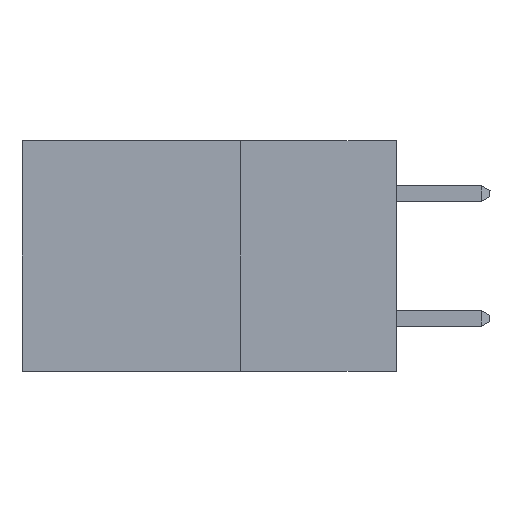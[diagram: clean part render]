
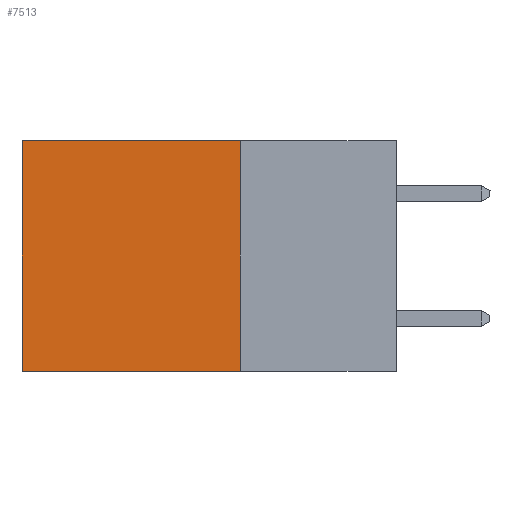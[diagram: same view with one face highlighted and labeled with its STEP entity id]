
A CAD part, left-side view. The second image highlights one B-rep face of the part: STEP entity #7513.
In plain terms, the highlighted planar face has unit normal (-1, 0, 0).
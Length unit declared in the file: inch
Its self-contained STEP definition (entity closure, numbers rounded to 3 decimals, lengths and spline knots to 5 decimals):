
#2 = CARTESIAN_POINT ( 'NONE',  ( 0.298, 0.25, 0. ) ) ;
#281 = FACE_OUTER_BOUND ( 'NONE', #5982, .T. ) ;
#2840 = LINE ( 'NONE', #5023, #15257 ) ;
#3210 = LINE ( 'NONE', #6717, #11351 ) ;
#3358 = ORIENTED_EDGE ( 'NONE', *, *, #16351, .T. ) ;
#3362 = EDGE_CURVE ( 'NONE', #13185, #14476, #3210, .T. ) ;
#3923 = VERTEX_POINT ( 'NONE', #6550 ) ;
#4254 = ORIENTED_EDGE ( 'NONE', *, *, #3362, .F. ) ;
#4864 = VECTOR ( 'NONE', #12818, 39.37008 ) ;
#4980 = ORIENTED_EDGE ( 'NONE', *, *, #13387, .T. ) ;
#5023 = CARTESIAN_POINT ( 'NONE',  ( 0.298, 0.25, 0. ) ) ;
#5630 = AXIS2_PLACEMENT_3D ( 'NONE', #13018, #17819, #8216 ) ;
#5639 = ORIENTED_EDGE ( 'NONE', *, *, #14670, .F. ) ;
#5982 = EDGE_LOOP ( 'NONE', ( #3358, #4254, #5639, #4980 ) ) ;
#6550 = CARTESIAN_POINT ( 'NONE',  ( 0.298, 0.25, 0. ) ) ;
#6600 = PLANE ( 'NONE',  #5630 ) ;
#6717 = CARTESIAN_POINT ( 'NONE',  ( 0.298, 0.25, -0.37 ) ) ;
#7513 = ADVANCED_FACE ( 'NONE', ( #281 ), #6600, .F. ) ;
#8216 = DIRECTION ( 'NONE',  ( 0., 0., -1. ) ) ;
#11351 = VECTOR ( 'NONE', #18877, 39.37008 ) ;
#11464 = DIRECTION ( 'NONE',  ( 0., 1., 0. ) ) ;
#12818 = DIRECTION ( 'NONE',  ( 0., 0., -1. ) ) ;
#13018 = CARTESIAN_POINT ( 'NONE',  ( 0.298, 0.25, 0. ) ) ;
#13185 = VERTEX_POINT ( 'NONE', #19055 ) ;
#13387 = EDGE_CURVE ( 'NONE', #3923, #14733, #2840, .T. ) ;
#13955 = LINE ( 'NONE', #2, #4864 ) ;
#14476 = VERTEX_POINT ( 'NONE', #18807 ) ;
#14572 = CARTESIAN_POINT ( 'NONE',  ( 0.298, 0.6, 0. ) ) ;
#14670 = EDGE_CURVE ( 'NONE', #3923, #13185, #13955, .T. ) ;
#14733 = VERTEX_POINT ( 'NONE', #19674 ) ;
#15257 = VECTOR ( 'NONE', #11464, 39.37008 ) ;
#16351 = EDGE_CURVE ( 'NONE', #14733, #14476, #18685, .T. ) ;
#17702 = VECTOR ( 'NONE', #20840, 39.37008 ) ;
#17819 = DIRECTION ( 'NONE',  ( 1., 0., 0. ) ) ;
#18685 = LINE ( 'NONE', #14572, #17702 ) ;
#18807 = CARTESIAN_POINT ( 'NONE',  ( 0.298, 0.6, -0.37 ) ) ;
#18877 = DIRECTION ( 'NONE',  ( 0., 1., 0. ) ) ;
#19055 = CARTESIAN_POINT ( 'NONE',  ( 0.298, 0.25, -0.37 ) ) ;
#19674 = CARTESIAN_POINT ( 'NONE',  ( 0.298, 0.6, 0. ) ) ;
#20840 = DIRECTION ( 'NONE',  ( 0., 0., -1. ) ) ;
